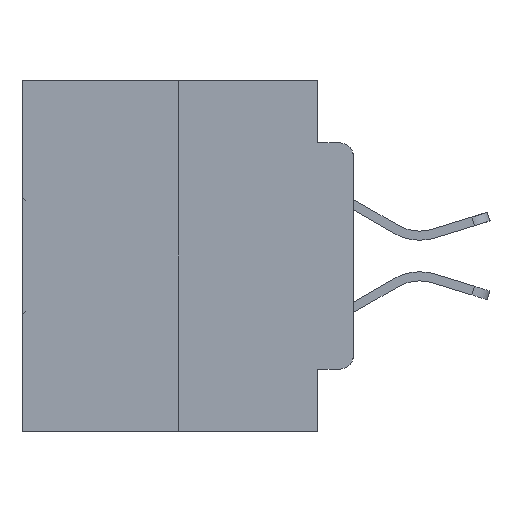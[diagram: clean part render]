
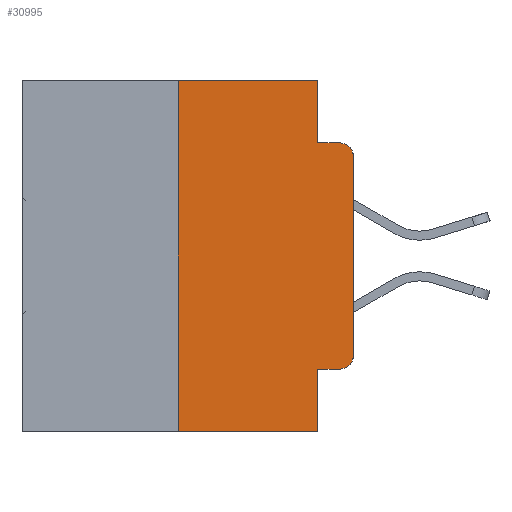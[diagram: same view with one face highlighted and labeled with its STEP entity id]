
A CAD part, left-side view. The second image highlights one B-rep face of the part: STEP entity #30995.
In plain terms, the highlighted planar face has unit normal (-1, 0, 0).
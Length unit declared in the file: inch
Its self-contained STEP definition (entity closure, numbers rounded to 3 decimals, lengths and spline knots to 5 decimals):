
#53 = EDGE_CURVE ( 'NONE', #4613, #6927, #14776, .T. ) ;
#638 = CARTESIAN_POINT ( 'NONE',  ( 0., 0.473, 0. ) ) ;
#643 = VERTEX_POINT ( 'NONE', #8830 ) ;
#768 = LINE ( 'NONE', #16117, #3585 ) ;
#812 = VECTOR ( 'NONE', #28773, 39.37008 ) ;
#845 = DIRECTION ( 'NONE',  ( 0., -1., 0. ) ) ;
#2310 = EDGE_CURVE ( 'NONE', #13305, #643, #14216, .T. ) ;
#2584 = ORIENTED_EDGE ( 'NONE', *, *, #21985, .T. ) ;
#3331 = DIRECTION ( 'NONE',  ( 1., 0., 0. ) ) ;
#3585 = VECTOR ( 'NONE', #30967, 39.37008 ) ;
#3753 = VERTEX_POINT ( 'NONE', #4975 ) ;
#3983 = DIRECTION ( 'NONE',  ( 0., -1., 0. ) ) ;
#4164 = CARTESIAN_POINT ( 'NONE',  ( 0., 0.473, 0. ) ) ;
#4613 = VERTEX_POINT ( 'NONE', #12827 ) ;
#4634 = VECTOR ( 'NONE', #19582, 39.37008 ) ;
#4738 = CARTESIAN_POINT ( 'NONE',  ( 0., 0.473, -0.5 ) ) ;
#4975 = CARTESIAN_POINT ( 'NONE',  ( 0., 0.051, 0. ) ) ;
#5223 = LINE ( 'NONE', #10786, #18438 ) ;
#5863 = LINE ( 'NONE', #21055, #812 ) ;
#6360 = DIRECTION ( 'NONE',  ( 0., 0., -1. ) ) ;
#6557 = VERTEX_POINT ( 'NONE', #22370 ) ;
#6927 = VERTEX_POINT ( 'NONE', #15482 ) ;
#8830 = CARTESIAN_POINT ( 'NONE',  ( 0., 0.02, -0.0885 ) ) ;
#8898 = LINE ( 'NONE', #4164, #9444 ) ;
#9444 = VECTOR ( 'NONE', #3983, 39.37008 ) ;
#9708 = VERTEX_POINT ( 'NONE', #15456 ) ;
#10070 = DIRECTION ( 'NONE',  ( 0., -1., 0. ) ) ;
#10618 = ORIENTED_EDGE ( 'NONE', *, *, #2310, .T. ) ;
#10739 = DIRECTION ( 'NONE',  ( 0., 0., -1. ) ) ;
#10786 = CARTESIAN_POINT ( 'NONE',  ( 0., 0.051, 0. ) ) ;
#11010 = AXIS2_PLACEMENT_3D ( 'NONE', #13275, #15282, #10739 ) ;
#11325 = EDGE_CURVE ( 'NONE', #6927, #13305, #14507, .T. ) ;
#12012 = EDGE_CURVE ( 'NONE', #6557, #29565, #768, .T. ) ;
#12773 = CARTESIAN_POINT ( 'NONE',  ( 0., 0., -0.1085 ) ) ;
#12827 = CARTESIAN_POINT ( 'NONE',  ( 0., 0.02, -0.4115 ) ) ;
#13275 = CARTESIAN_POINT ( 'NONE',  ( 0., 0.02, -0.3915 ) ) ;
#13305 = VERTEX_POINT ( 'NONE', #12773 ) ;
#13695 = DIRECTION ( 'NONE',  ( 0., 0., -1. ) ) ;
#14216 = CIRCLE ( 'NONE', #16919, 0.02 ) ;
#14328 = CARTESIAN_POINT ( 'NONE',  ( 0., 0.25, 0. ) ) ;
#14507 = LINE ( 'NONE', #24795, #4634 ) ;
#14577 = ORIENTED_EDGE ( 'NONE', *, *, #11325, .T. ) ;
#14776 = CIRCLE ( 'NONE', #11010, 0.02 ) ;
#15282 = DIRECTION ( 'NONE',  ( -1., 0., 0. ) ) ;
#15440 = VERTEX_POINT ( 'NONE', #21106 ) ;
#15456 = CARTESIAN_POINT ( 'NONE',  ( 0., 0.051, -0.5 ) ) ;
#15482 = CARTESIAN_POINT ( 'NONE',  ( 0., 0., -0.3915 ) ) ;
#16117 = CARTESIAN_POINT ( 'NONE',  ( 0., 0.25, 0. ) ) ;
#16158 = PLANE ( 'NONE',  #30442 ) ;
#16919 = AXIS2_PLACEMENT_3D ( 'NONE', #26825, #29021, #13695 ) ;
#17149 = ORIENTED_EDGE ( 'NONE', *, *, #29458, .T. ) ;
#17482 = CARTESIAN_POINT ( 'NONE',  ( 0., 0.051, -0.4115 ) ) ;
#17538 = EDGE_CURVE ( 'NONE', #15440, #643, #31303, .T. ) ;
#18407 = CARTESIAN_POINT ( 'NONE',  ( 0., 0.051, -0.4115 ) ) ;
#18438 = VECTOR ( 'NONE', #6360, 39.37008 ) ;
#18530 = DIRECTION ( 'NONE',  ( 0., 0., -1. ) ) ;
#19582 = DIRECTION ( 'NONE',  ( 0., 0., 1. ) ) ;
#20804 = EDGE_CURVE ( 'NONE', #26072, #9708, #5223, .T. ) ;
#21055 = CARTESIAN_POINT ( 'NONE',  ( 0., 0.051, 0. ) ) ;
#21106 = CARTESIAN_POINT ( 'NONE',  ( 0., 0.051, -0.0885 ) ) ;
#21985 = EDGE_CURVE ( 'NONE', #6557, #9708, #25305, .T. ) ;
#22370 = CARTESIAN_POINT ( 'NONE',  ( 0., 0.25, -0.5 ) ) ;
#22461 = ORIENTED_EDGE ( 'NONE', *, *, #27302, .F. ) ;
#23244 = VECTOR ( 'NONE', #33204, 39.37008 ) ;
#23589 = FACE_OUTER_BOUND ( 'NONE', #32782, .T. ) ;
#23738 = VECTOR ( 'NONE', #10070, 39.37008 ) ;
#24795 = CARTESIAN_POINT ( 'NONE',  ( 0., 0., 0. ) ) ;
#25305 = LINE ( 'NONE', #4738, #23244 ) ;
#25869 = EDGE_CURVE ( 'NONE', #3753, #15440, #5863, .T. ) ;
#26072 = VERTEX_POINT ( 'NONE', #17482 ) ;
#26825 = CARTESIAN_POINT ( 'NONE',  ( 0., 0.02, -0.1085 ) ) ;
#27302 = EDGE_CURVE ( 'NONE', #29565, #3753, #8898, .T. ) ;
#28094 = CARTESIAN_POINT ( 'NONE',  ( 0., 0.051, -0.0885 ) ) ;
#28753 = ORIENTED_EDGE ( 'NONE', *, *, #17538, .F. ) ;
#28773 = DIRECTION ( 'NONE',  ( 0., 0., -1. ) ) ;
#28995 = LINE ( 'NONE', #18407, #32709 ) ;
#29021 = DIRECTION ( 'NONE',  ( -1., 0., 0. ) ) ;
#29458 = EDGE_CURVE ( 'NONE', #26072, #4613, #28995, .T. ) ;
#29565 = VERTEX_POINT ( 'NONE', #14328 ) ;
#30442 = AXIS2_PLACEMENT_3D ( 'NONE', #638, #3331, #18530 ) ;
#30967 = DIRECTION ( 'NONE',  ( 0., 0., 1. ) ) ;
#30995 = ADVANCED_FACE ( 'NONE', ( #23589 ), #16158, .F. ) ;
#31303 = LINE ( 'NONE', #28094, #23738 ) ;
#32138 = ORIENTED_EDGE ( 'NONE', *, *, #53, .T. ) ;
#32195 = ORIENTED_EDGE ( 'NONE', *, *, #25869, .F. ) ;
#32262 = ORIENTED_EDGE ( 'NONE', *, *, #12012, .F. ) ;
#32709 = VECTOR ( 'NONE', #845, 39.37008 ) ;
#32782 = EDGE_LOOP ( 'NONE', ( #14577, #10618, #28753, #32195, #22461, #32262, #2584, #32988, #17149, #32138 ) ) ;
#32988 = ORIENTED_EDGE ( 'NONE', *, *, #20804, .F. ) ;
#33204 = DIRECTION ( 'NONE',  ( 0., -1., 0. ) ) ;
